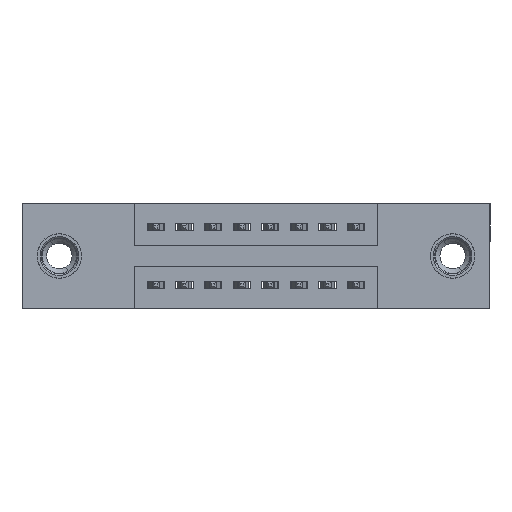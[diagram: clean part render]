
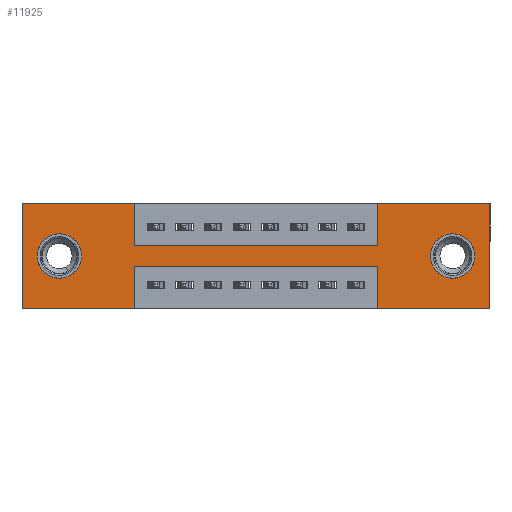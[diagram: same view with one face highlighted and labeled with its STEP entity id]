
A CAD part, front view. The second image highlights one B-rep face of the part: STEP entity #11925.
In plain terms, the highlighted planar face has unit normal (0, -1, 0).
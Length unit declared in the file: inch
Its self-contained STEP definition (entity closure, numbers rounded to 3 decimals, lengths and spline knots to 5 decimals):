
#3 = LINE ( 'NONE', #1745, #4999 ) ;
#25 = CARTESIAN_POINT ( 'NONE',  ( 0.3925, 0., -0.22 ) ) ;
#153 = CIRCLE ( 'NONE', #3730, 0.078 ) ;
#155 = EDGE_CURVE ( 'NONE', #11530, #8668, #1275, .T. ) ;
#178 = ORIENTED_EDGE ( 'NONE', *, *, #10319, .T. ) ;
#203 = LINE ( 'NONE', #5816, #7854 ) ;
#226 = VERTEX_POINT ( 'NONE', #12789 ) ;
#231 = DIRECTION ( 'NONE',  ( 1., 0., 0. ) ) ;
#240 = ORIENTED_EDGE ( 'NONE', *, *, #1463, .F. ) ;
#334 = DIRECTION ( 'NONE',  ( -1., 0., 0. ) ) ;
#504 = LINE ( 'NONE', #10065, #7699 ) ;
#596 = DIRECTION ( 'NONE',  ( 0., 1., 0. ) ) ;
#603 = ORIENTED_EDGE ( 'NONE', *, *, #7805, .F. ) ;
#715 = EDGE_CURVE ( 'NONE', #2933, #1129, #153, .T. ) ;
#803 = DIRECTION ( 'NONE',  ( 1., 0., 0. ) ) ;
#1083 = AXIS2_PLACEMENT_3D ( 'NONE', #4893, #5884, #3848 ) ;
#1129 = VERTEX_POINT ( 'NONE', #3199 ) ;
#1275 = LINE ( 'NONE', #5563, #7345 ) ;
#1283 = ORIENTED_EDGE ( 'NONE', *, *, #8112, .F. ) ;
#1330 = CARTESIAN_POINT ( 'NONE',  ( 0.3925, 0., 0. ) ) ;
#1370 = EDGE_CURVE ( 'NONE', #12199, #10441, #6987, .T. ) ;
#1463 = EDGE_CURVE ( 'NONE', #9977, #9764, #4038, .T. ) ;
#1488 = ORIENTED_EDGE ( 'NONE', *, *, #10422, .F. ) ;
#1499 = CARTESIAN_POINT ( 'NONE',  ( 1.635, 0., 0. ) ) ;
#1569 = LINE ( 'NONE', #2318, #1726 ) ;
#1642 = ORIENTED_EDGE ( 'NONE', *, *, #11106, .F. ) ;
#1726 = VECTOR ( 'NONE', #10401, 39.37008 ) ;
#1745 = CARTESIAN_POINT ( 'NONE',  ( 0., 0., -0.37 ) ) ;
#1762 = DIRECTION ( 'NONE',  ( 0., 0., -1. ) ) ;
#2073 = CARTESIAN_POINT ( 'NONE',  ( 1.635, 0., -0.37 ) ) ;
#2190 = FACE_OUTER_BOUND ( 'NONE', #10785, .T. ) ;
#2207 = EDGE_LOOP ( 'NONE', ( #3974, #178 ) ) ;
#2318 = CARTESIAN_POINT ( 'NONE',  ( 1.635, 0., 0. ) ) ;
#2330 = VERTEX_POINT ( 'NONE', #9948 ) ;
#2438 = CARTESIAN_POINT ( 'NONE',  ( 1.505, 0., -0.107 ) ) ;
#2439 = DIRECTION ( 'NONE',  ( 0., 0., -1. ) ) ;
#2643 = VERTEX_POINT ( 'NONE', #9815 ) ;
#2667 = LINE ( 'NONE', #25, #11343 ) ;
#2744 = EDGE_CURVE ( 'NONE', #2643, #3295, #10800, .T. ) ;
#2823 = CIRCLE ( 'NONE', #1083, 0.078 ) ;
#2933 = VERTEX_POINT ( 'NONE', #2438 ) ;
#2958 = VECTOR ( 'NONE', #4687, 39.37008 ) ;
#3040 = CARTESIAN_POINT ( 'NONE',  ( 0., 0., -0.37 ) ) ;
#3199 = CARTESIAN_POINT ( 'NONE',  ( 1.505, 0., -0.263 ) ) ;
#3264 = VERTEX_POINT ( 'NONE', #2073 ) ;
#3295 = VERTEX_POINT ( 'NONE', #5949 ) ;
#3317 = ORIENTED_EDGE ( 'NONE', *, *, #2744, .F. ) ;
#3340 = LINE ( 'NONE', #11171, #12972 ) ;
#3425 = VECTOR ( 'NONE', #12094, 39.37008 ) ;
#3730 = AXIS2_PLACEMENT_3D ( 'NONE', #6672, #596, #10736 ) ;
#3756 = CARTESIAN_POINT ( 'NONE',  ( 1.505, 0., -0.185 ) ) ;
#3790 = VERTEX_POINT ( 'NONE', #10827 ) ;
#3822 = DIRECTION ( 'NONE',  ( 1., 0., 0. ) ) ;
#3848 = DIRECTION ( 'NONE',  ( 0., 0., 1. ) ) ;
#3974 = ORIENTED_EDGE ( 'NONE', *, *, #715, .T. ) ;
#4028 = PLANE ( 'NONE',  #11381 ) ;
#4038 = LINE ( 'NONE', #10674, #2958 ) ;
#4296 = EDGE_CURVE ( 'NONE', #3295, #4646, #10923, .T. ) ;
#4483 = CARTESIAN_POINT ( 'NONE',  ( 0.13, 0., -0.185 ) ) ;
#4646 = VERTEX_POINT ( 'NONE', #1499 ) ;
#4687 = DIRECTION ( 'NONE',  ( 0., 0., -1. ) ) ;
#4827 = ORIENTED_EDGE ( 'NONE', *, *, #5492, .F. ) ;
#4893 = CARTESIAN_POINT ( 'NONE',  ( 0.13, 0., -0.185 ) ) ;
#4999 = VECTOR ( 'NONE', #8681, 39.37008 ) ;
#5103 = CARTESIAN_POINT ( 'NONE',  ( 0., 0., 0. ) ) ;
#5237 = VECTOR ( 'NONE', #3822, 39.37008 ) ;
#5492 = EDGE_CURVE ( 'NONE', #226, #11010, #9451, .T. ) ;
#5499 = CARTESIAN_POINT ( 'NONE',  ( 0.13, 0., -0.263 ) ) ;
#5525 = ORIENTED_EDGE ( 'NONE', *, *, #6589, .F. ) ;
#5563 = CARTESIAN_POINT ( 'NONE',  ( 0.3925, 0., 0. ) ) ;
#5652 = AXIS2_PLACEMENT_3D ( 'NONE', #3756, #6767, #1762 ) ;
#5717 = CARTESIAN_POINT ( 'NONE',  ( 0., 0., 0. ) ) ;
#5816 = CARTESIAN_POINT ( 'NONE',  ( 0., 0., 0. ) ) ;
#5880 = CARTESIAN_POINT ( 'NONE',  ( 0.13, 0., -0.107 ) ) ;
#5884 = DIRECTION ( 'NONE',  ( 0., 1., 0. ) ) ;
#5949 = CARTESIAN_POINT ( 'NONE',  ( 1.2425, 0., 0. ) ) ;
#5983 = DIRECTION ( 'NONE',  ( 0., 0., -1. ) ) ;
#6091 = FACE_BOUND ( 'NONE', #10686, .T. ) ;
#6516 = DIRECTION ( 'NONE',  ( 0., 0., 1. ) ) ;
#6589 = EDGE_CURVE ( 'NONE', #11010, #11530, #203, .T. ) ;
#6592 = LINE ( 'NONE', #12255, #12150 ) ;
#6664 = ORIENTED_EDGE ( 'NONE', *, *, #11795, .T. ) ;
#6672 = CARTESIAN_POINT ( 'NONE',  ( 1.505, 0., -0.185 ) ) ;
#6750 = ORIENTED_EDGE ( 'NONE', *, *, #9363, .F. ) ;
#6767 = DIRECTION ( 'NONE',  ( 0., 1., 0. ) ) ;
#6987 = CIRCLE ( 'NONE', #8347, 0.078 ) ;
#7016 = FACE_BOUND ( 'NONE', #2207, .T. ) ;
#7174 = ORIENTED_EDGE ( 'NONE', *, *, #155, .F. ) ;
#7345 = VECTOR ( 'NONE', #2439, 39.37008 ) ;
#7596 = DIRECTION ( 'NONE',  ( 0., 0., 1. ) ) ;
#7699 = VECTOR ( 'NONE', #10922, 39.37008 ) ;
#7805 = EDGE_CURVE ( 'NONE', #9764, #226, #3, .T. ) ;
#7854 = VECTOR ( 'NONE', #803, 39.37008 ) ;
#8112 = EDGE_CURVE ( 'NONE', #4646, #3264, #1569, .T. ) ;
#8347 = AXIS2_PLACEMENT_3D ( 'NONE', #4483, #8376, #6516 ) ;
#8376 = DIRECTION ( 'NONE',  ( 0., 1., 0. ) ) ;
#8668 = VERTEX_POINT ( 'NONE', #12608 ) ;
#8681 = DIRECTION ( 'NONE',  ( -1., 0., 0. ) ) ;
#9028 = DIRECTION ( 'NONE',  ( 0., 0., 1. ) ) ;
#9187 = DIRECTION ( 'NONE',  ( 0., -1., 0. ) ) ;
#9217 = EDGE_CURVE ( 'NONE', #8668, #2643, #6592, .T. ) ;
#9363 = EDGE_CURVE ( 'NONE', #2330, #3790, #3340, .T. ) ;
#9451 = LINE ( 'NONE', #12692, #12510 ) ;
#9719 = ORIENTED_EDGE ( 'NONE', *, *, #4296, .F. ) ;
#9764 = VERTEX_POINT ( 'NONE', #10850 ) ;
#9815 = CARTESIAN_POINT ( 'NONE',  ( 1.2425, 0., -0.15 ) ) ;
#9948 = CARTESIAN_POINT ( 'NONE',  ( 1.2425, 0., -0.37 ) ) ;
#9977 = VERTEX_POINT ( 'NONE', #12027 ) ;
#10065 = CARTESIAN_POINT ( 'NONE',  ( 0., 0., -0.37 ) ) ;
#10319 = EDGE_CURVE ( 'NONE', #1129, #2933, #10543, .T. ) ;
#10401 = DIRECTION ( 'NONE',  ( 0., 0., -1. ) ) ;
#10422 = EDGE_CURVE ( 'NONE', #3264, #2330, #504, .T. ) ;
#10441 = VERTEX_POINT ( 'NONE', #5880 ) ;
#10543 = CIRCLE ( 'NONE', #5652, 0.078 ) ;
#10674 = CARTESIAN_POINT ( 'NONE',  ( 0.3925, 0., -0.37 ) ) ;
#10686 = EDGE_LOOP ( 'NONE', ( #6664, #10733 ) ) ;
#10733 = ORIENTED_EDGE ( 'NONE', *, *, #1370, .T. ) ;
#10736 = DIRECTION ( 'NONE',  ( 0., 0., -1. ) ) ;
#10785 = EDGE_LOOP ( 'NONE', ( #240, #1642, #6750, #1488, #1283, #9719, #3317, #12434, #7174, #5525, #4827, #603 ) ) ;
#10800 = LINE ( 'NONE', #11061, #3425 ) ;
#10827 = CARTESIAN_POINT ( 'NONE',  ( 1.2425, 0., -0.22 ) ) ;
#10850 = CARTESIAN_POINT ( 'NONE',  ( 0.3925, 0., -0.37 ) ) ;
#10922 = DIRECTION ( 'NONE',  ( -1., 0., 0. ) ) ;
#10923 = LINE ( 'NONE', #5717, #5237 ) ;
#11010 = VERTEX_POINT ( 'NONE', #5103 ) ;
#11061 = CARTESIAN_POINT ( 'NONE',  ( 1.2425, 0., 0. ) ) ;
#11106 = EDGE_CURVE ( 'NONE', #3790, #9977, #2667, .T. ) ;
#11171 = CARTESIAN_POINT ( 'NONE',  ( 1.2425, 0., -0.37 ) ) ;
#11343 = VECTOR ( 'NONE', #334, 39.37008 ) ;
#11381 = AXIS2_PLACEMENT_3D ( 'NONE', #3040, #9187, #5983 ) ;
#11530 = VERTEX_POINT ( 'NONE', #1330 ) ;
#11795 = EDGE_CURVE ( 'NONE', #10441, #12199, #2823, .T. ) ;
#11925 = ADVANCED_FACE ( 'NONE', ( #7016, #6091, #2190 ), #4028, .T. ) ;
#12027 = CARTESIAN_POINT ( 'NONE',  ( 0.3925, 0., -0.22 ) ) ;
#12094 = DIRECTION ( 'NONE',  ( 0., 0., 1. ) ) ;
#12150 = VECTOR ( 'NONE', #231, 39.37008 ) ;
#12199 = VERTEX_POINT ( 'NONE', #5499 ) ;
#12255 = CARTESIAN_POINT ( 'NONE',  ( 0.3925, 0., -0.15 ) ) ;
#12434 = ORIENTED_EDGE ( 'NONE', *, *, #9217, .F. ) ;
#12510 = VECTOR ( 'NONE', #7596, 39.37008 ) ;
#12608 = CARTESIAN_POINT ( 'NONE',  ( 0.3925, 0., -0.15 ) ) ;
#12692 = CARTESIAN_POINT ( 'NONE',  ( 0., 0., 0. ) ) ;
#12789 = CARTESIAN_POINT ( 'NONE',  ( 0., 0., -0.37 ) ) ;
#12972 = VECTOR ( 'NONE', #9028, 39.37008 ) ;
